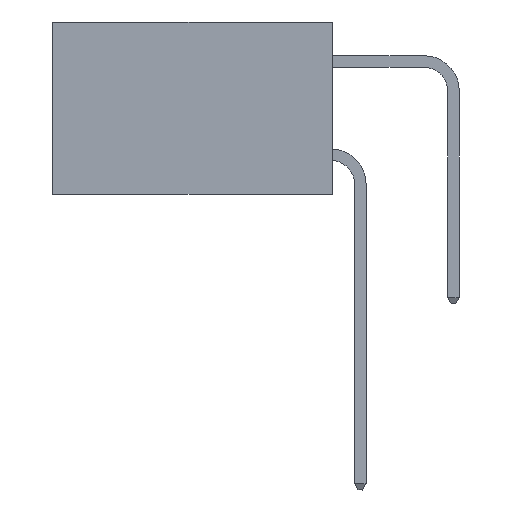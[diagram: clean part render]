
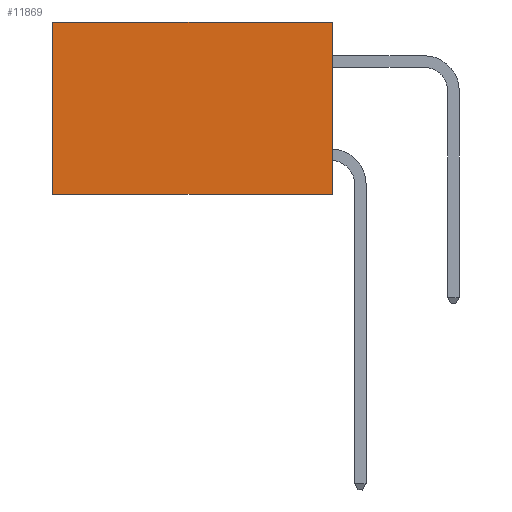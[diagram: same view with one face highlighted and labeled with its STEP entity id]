
A CAD part, left-side view. The second image highlights one B-rep face of the part: STEP entity #11869.
In plain terms, the highlighted planar face has unit normal (-1, 0, 0).
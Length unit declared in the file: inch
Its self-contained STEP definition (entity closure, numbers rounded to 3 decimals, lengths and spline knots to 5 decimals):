
#407 = CARTESIAN_POINT ( 'NONE',  ( 0.2615, 0., 0. ) ) ;
#599 = DIRECTION ( 'NONE',  ( 1., 0., 0. ) ) ;
#812 = VECTOR ( 'NONE', #3076, 39.37008 ) ;
#935 = ORIENTED_EDGE ( 'NONE', *, *, #9194, .F. ) ;
#1434 = LINE ( 'NONE', #7199, #10364 ) ;
#2419 = ORIENTED_EDGE ( 'NONE', *, *, #2648, .F. ) ;
#2648 = EDGE_CURVE ( 'NONE', #5367, #9123, #4214, .T. ) ;
#2738 = VERTEX_POINT ( 'NONE', #3365 ) ;
#3076 = DIRECTION ( 'NONE',  ( 0., 0., -1. ) ) ;
#3133 = ORIENTED_EDGE ( 'NONE', *, *, #7484, .T. ) ;
#3234 = CARTESIAN_POINT ( 'NONE',  ( 0.2615, 0.6, -0.37 ) ) ;
#3365 = CARTESIAN_POINT ( 'NONE',  ( 0.2615, 0.6, 0. ) ) ;
#3665 = DIRECTION ( 'NONE',  ( 0., 1., 0. ) ) ;
#3737 = EDGE_LOOP ( 'NONE', ( #12297, #2419, #935, #3133 ) ) ;
#4214 = LINE ( 'NONE', #8832, #10480 ) ;
#4452 = VECTOR ( 'NONE', #8347, 39.37008 ) ;
#5367 = VERTEX_POINT ( 'NONE', #11378 ) ;
#7199 = CARTESIAN_POINT ( 'NONE',  ( 0.2615, 0., 0. ) ) ;
#7484 = EDGE_CURVE ( 'NONE', #9319, #2738, #1434, .T. ) ;
#8347 = DIRECTION ( 'NONE',  ( 0., 0., -1. ) ) ;
#8494 = CARTESIAN_POINT ( 'NONE',  ( 0.2615, 0., -0.37 ) ) ;
#8832 = CARTESIAN_POINT ( 'NONE',  ( 0.2615, 0., -0.37 ) ) ;
#9123 = VERTEX_POINT ( 'NONE', #12415 ) ;
#9194 = EDGE_CURVE ( 'NONE', #9319, #5367, #11866, .T. ) ;
#9319 = VERTEX_POINT ( 'NONE', #407 ) ;
#9771 = PLANE ( 'NONE',  #12844 ) ;
#10364 = VECTOR ( 'NONE', #3665, 39.37008 ) ;
#10480 = VECTOR ( 'NONE', #12344, 39.37008 ) ;
#10910 = FACE_OUTER_BOUND ( 'NONE', #3737, .T. ) ;
#11134 = CARTESIAN_POINT ( 'NONE',  ( 0.2615, 0., -0.37 ) ) ;
#11228 = LINE ( 'NONE', #3234, #812 ) ;
#11378 = CARTESIAN_POINT ( 'NONE',  ( 0.2615, 0., -0.37 ) ) ;
#11451 = EDGE_CURVE ( 'NONE', #2738, #9123, #11228, .T. ) ;
#11866 = LINE ( 'NONE', #8494, #4452 ) ;
#11869 = ADVANCED_FACE ( 'NONE', ( #10910 ), #9771, .F. ) ;
#12297 = ORIENTED_EDGE ( 'NONE', *, *, #11451, .T. ) ;
#12344 = DIRECTION ( 'NONE',  ( 0., 1., 0. ) ) ;
#12415 = CARTESIAN_POINT ( 'NONE',  ( 0.2615, 0.6, -0.37 ) ) ;
#12844 = AXIS2_PLACEMENT_3D ( 'NONE', #11134, #599, #14444 ) ;
#14444 = DIRECTION ( 'NONE',  ( 0., 0., -1. ) ) ;
